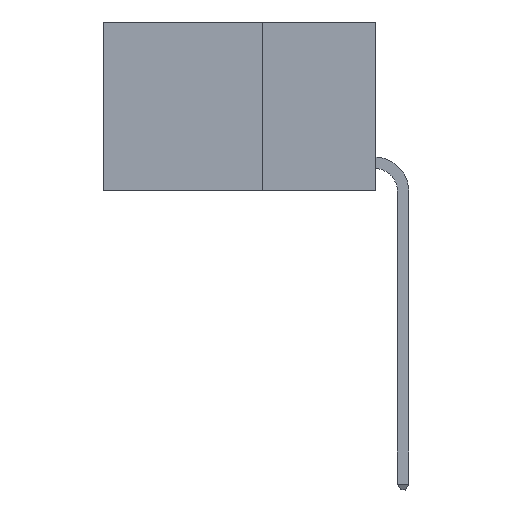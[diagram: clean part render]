
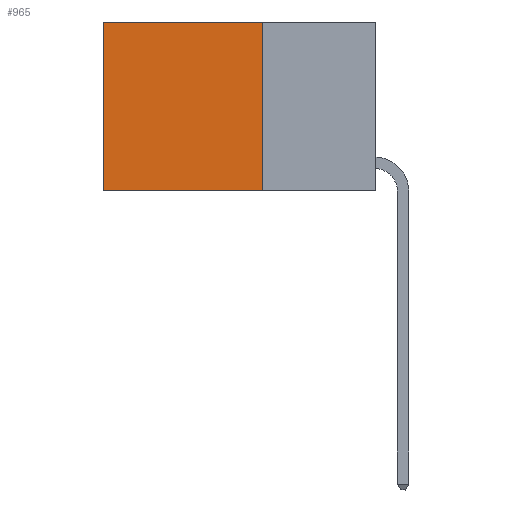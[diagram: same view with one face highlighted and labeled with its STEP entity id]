
A CAD part, left-side view. The second image highlights one B-rep face of the part: STEP entity #965.
In plain terms, the highlighted planar face has unit normal (-1, 0, 0).
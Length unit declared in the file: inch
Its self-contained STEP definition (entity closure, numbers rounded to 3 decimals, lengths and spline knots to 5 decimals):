
#382 = CARTESIAN_POINT ( 'NONE',  ( 0.2625, 0.25, 0. ) ) ;
#856 = VERTEX_POINT ( 'NONE', #12723 ) ;
#965 = ADVANCED_FACE ( 'NONE', ( #2741 ), #7195, .F. ) ;
#1653 = VERTEX_POINT ( 'NONE', #2873 ) ;
#1891 = LINE ( 'NONE', #12310, #14113 ) ;
#2658 = VERTEX_POINT ( 'NONE', #10841 ) ;
#2741 = FACE_OUTER_BOUND ( 'NONE', #13183, .T. ) ;
#2873 = CARTESIAN_POINT ( 'NONE',  ( 0.2625, 0.6, 0. ) ) ;
#3573 = CARTESIAN_POINT ( 'NONE',  ( 0.2625, 0.6, 0. ) ) ;
#3880 = CARTESIAN_POINT ( 'NONE',  ( 0.2625, 0.25, 0. ) ) ;
#4036 = DIRECTION ( 'NONE',  ( 0., 1., 0. ) ) ;
#4082 = VECTOR ( 'NONE', #13224, 39.37008 ) ;
#4520 = ORIENTED_EDGE ( 'NONE', *, *, #12521, .T. ) ;
#4704 = DIRECTION ( 'NONE',  ( 0., 0., -1. ) ) ;
#4793 = VERTEX_POINT ( 'NONE', #8527 ) ;
#6214 = DIRECTION ( 'NONE',  ( 0., 0., -1. ) ) ;
#6292 = LINE ( 'NONE', #10913, #6737 ) ;
#6737 = VECTOR ( 'NONE', #4036, 39.37008 ) ;
#7195 = PLANE ( 'NONE',  #14373 ) ;
#8417 = EDGE_CURVE ( 'NONE', #4793, #2658, #1891, .T. ) ;
#8527 = CARTESIAN_POINT ( 'NONE',  ( 0.2625, 0.25, 0. ) ) ;
#8684 = ORIENTED_EDGE ( 'NONE', *, *, #13600, .T. ) ;
#9340 = VECTOR ( 'NONE', #4704, 39.37008 ) ;
#9526 = LINE ( 'NONE', #3573, #9340 ) ;
#9732 = ORIENTED_EDGE ( 'NONE', *, *, #13989, .F. ) ;
#9793 = ORIENTED_EDGE ( 'NONE', *, *, #8417, .F. ) ;
#9802 = DIRECTION ( 'NONE',  ( 0., 0., -1. ) ) ;
#10595 = DIRECTION ( 'NONE',  ( 1., 0., 0. ) ) ;
#10841 = CARTESIAN_POINT ( 'NONE',  ( 0.2625, 0.25, -0.37 ) ) ;
#10913 = CARTESIAN_POINT ( 'NONE',  ( 0.2625, 0.25, -0.37 ) ) ;
#12310 = CARTESIAN_POINT ( 'NONE',  ( 0.2625, 0.25, 0. ) ) ;
#12521 = EDGE_CURVE ( 'NONE', #1653, #856, #9526, .T. ) ;
#12723 = CARTESIAN_POINT ( 'NONE',  ( 0.2625, 0.6, -0.37 ) ) ;
#13183 = EDGE_LOOP ( 'NONE', ( #4520, #9732, #9793, #8684 ) ) ;
#13224 = DIRECTION ( 'NONE',  ( 0., 1., 0. ) ) ;
#13600 = EDGE_CURVE ( 'NONE', #4793, #1653, #14347, .T. ) ;
#13989 = EDGE_CURVE ( 'NONE', #2658, #856, #6292, .T. ) ;
#14113 = VECTOR ( 'NONE', #9802, 39.37008 ) ;
#14347 = LINE ( 'NONE', #382, #4082 ) ;
#14373 = AXIS2_PLACEMENT_3D ( 'NONE', #3880, #10595, #6214 ) ;
